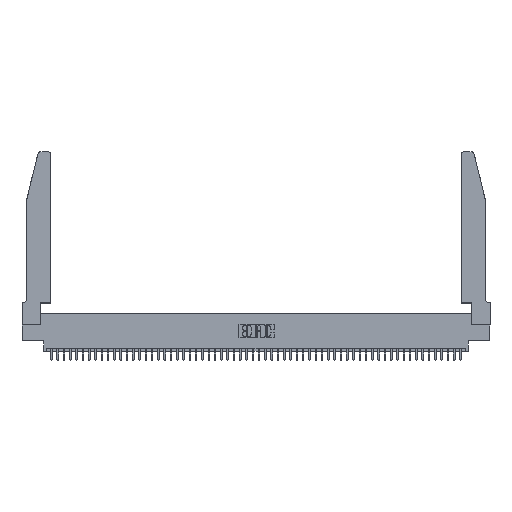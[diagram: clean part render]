
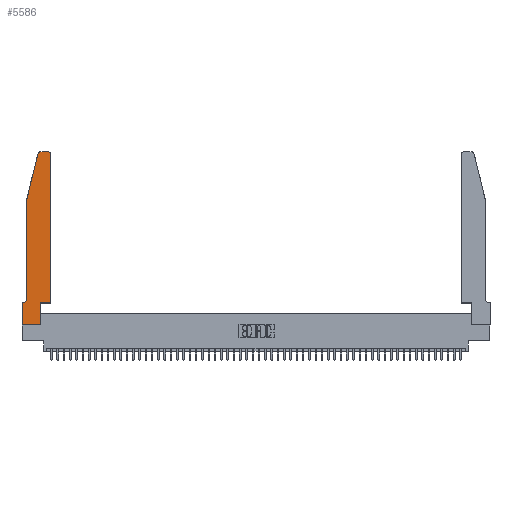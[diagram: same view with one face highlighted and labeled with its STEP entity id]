
A CAD part, top view. The second image highlights one B-rep face of the part: STEP entity #5586.
In plain terms, the highlighted planar face has unit normal (0, 0, 1).
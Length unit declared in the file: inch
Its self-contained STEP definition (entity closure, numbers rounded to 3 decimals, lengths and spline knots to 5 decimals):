
#58 = DIRECTION ( 'NONE',  ( 0., 0., 1. ) ) ;
#455 = VECTOR ( 'NONE', #43000, 39.37008 ) ;
#641 = VERTEX_POINT ( 'NONE', #29714 ) ;
#817 = CARTESIAN_POINT ( 'NONE',  ( 0.0755, 2., 0.37 ) ) ;
#2398 = EDGE_CURVE ( 'NONE', #641, #36479, #14091, .T. ) ;
#4239 = CARTESIAN_POINT ( 'NONE',  ( 0.0755, 2., 0.37 ) ) ;
#4984 = ORIENTED_EDGE ( 'NONE', *, *, #37938, .T. ) ;
#5417 = VERTEX_POINT ( 'NONE', #32110 ) ;
#5586 = ADVANCED_FACE ( 'NONE', ( #47401 ), #8247, .T. ) ;
#5606 = VERTEX_POINT ( 'NONE', #4239 ) ;
#5927 = ORIENTED_EDGE ( 'NONE', *, *, #8302, .T. ) ;
#6263 = VERTEX_POINT ( 'NONE', #37422 ) ;
#6412 = DIRECTION ( 'NONE',  ( 0., -1., 0. ) ) ;
#7807 = VECTOR ( 'NONE', #10816, 39.37008 ) ;
#8247 = PLANE ( 'NONE',  #50703 ) ;
#8302 = EDGE_CURVE ( 'NONE', #5606, #12480, #20822, .T. ) ;
#8581 = EDGE_CURVE ( 'NONE', #42707, #641, #31118, .T. ) ;
#9226 = VECTOR ( 'NONE', #50656, 39.37008 ) ;
#10210 = DIRECTION ( 'NONE',  ( 0., 0., -1. ) ) ;
#10615 = CARTESIAN_POINT ( 'NONE',  ( 0.0755, 0.42, 0.37 ) ) ;
#10816 = DIRECTION ( 'NONE',  ( 1., 0., 0. ) ) ;
#12480 = VERTEX_POINT ( 'NONE', #10615 ) ;
#13121 = CARTESIAN_POINT ( 'NONE',  ( 0.0755, 0.35, 0.37 ) ) ;
#13303 = CARTESIAN_POINT ( 'NONE',  ( 0.2865, 0.35, 0.37 ) ) ;
#13602 = EDGE_LOOP ( 'NONE', ( #52687, #4984, #48419, #5927, #28442, #44120, #22112, #52174, #36251, #24450, #34792, #44723 ) ) ;
#14091 = LINE ( 'NONE', #51625, #45785 ) ;
#14487 = DIRECTION ( 'NONE',  ( 0., 1., 0. ) ) ;
#14609 = VERTEX_POINT ( 'NONE', #30704 ) ;
#15669 = EDGE_CURVE ( 'NONE', #36479, #23356, #40565, .T. ) ;
#17044 = CARTESIAN_POINT ( 'NONE',  ( 0.0755, 2., 0.37 ) ) ;
#17643 = EDGE_CURVE ( 'NONE', #41685, #5606, #53184, .T. ) ;
#18992 = EDGE_CURVE ( 'NONE', #5417, #22556, #51760, .T. ) ;
#20329 = VECTOR ( 'NONE', #21215, 39.37008 ) ;
#20747 = CARTESIAN_POINT ( 'NONE',  ( 0., 0.35, 0.37 ) ) ;
#20822 = LINE ( 'NONE', #817, #31774 ) ;
#20905 = CARTESIAN_POINT ( 'NONE',  ( 0.25487, 2.72718, 0.37 ) ) ;
#20945 = CARTESIAN_POINT ( 'NONE',  ( 0.284, 2.72, 0.37 ) ) ;
#21215 = DIRECTION ( 'NONE',  ( -0.239, -0.971, 0. ) ) ;
#21422 = DIRECTION ( 'NONE',  ( 0., 0., 1. ) ) ;
#21549 = LINE ( 'NONE', #46560, #9226 ) ;
#22112 = ORIENTED_EDGE ( 'NONE', *, *, #18992, .T. ) ;
#22556 = VERTEX_POINT ( 'NONE', #28839 ) ;
#22835 = CARTESIAN_POINT ( 'NONE',  ( 0.4505, 2.72, 0.37 ) ) ;
#22876 = EDGE_CURVE ( 'NONE', #12480, #6263, #52222, .T. ) ;
#23356 = VERTEX_POINT ( 'NONE', #46453 ) ;
#23454 = EDGE_CURVE ( 'NONE', #23356, #14609, #33487, .T. ) ;
#24450 = ORIENTED_EDGE ( 'NONE', *, *, #8581, .T. ) ;
#25080 = DIRECTION ( 'NONE',  ( 1., 0., 0. ) ) ;
#27059 = VECTOR ( 'NONE', #46171, 39.37008 ) ;
#27079 = EDGE_CURVE ( 'NONE', #22556, #49435, #21549, .T. ) ;
#27228 = CARTESIAN_POINT ( 'NONE',  ( 0., 0., 0.37 ) ) ;
#27248 = CARTESIAN_POINT ( 'NONE',  ( 0.4505, 0.35, 0.37 ) ) ;
#28441 = DIRECTION ( 'NONE',  ( 0., 1., 0. ) ) ;
#28442 = ORIENTED_EDGE ( 'NONE', *, *, #22876, .T. ) ;
#28558 = VECTOR ( 'NONE', #6412, 39.37008 ) ;
#28839 = CARTESIAN_POINT ( 'NONE',  ( 0., 0., 0.37 ) ) ;
#29033 = DIRECTION ( 'NONE',  ( 1., 0., 0. ) ) ;
#29714 = CARTESIAN_POINT ( 'NONE',  ( 0.4505, 0.35, 0.37 ) ) ;
#29892 = LINE ( 'NONE', #40903, #43458 ) ;
#30704 = CARTESIAN_POINT ( 'NONE',  ( 0.284, 2.75, 0.37 ) ) ;
#31118 = LINE ( 'NONE', #27248, #7807 ) ;
#31774 = VECTOR ( 'NONE', #37888, 39.37008 ) ;
#32110 = CARTESIAN_POINT ( 'NONE',  ( 0., 0.35, 0.37 ) ) ;
#32181 = EDGE_CURVE ( 'NONE', #6263, #5417, #48984, .T. ) ;
#32768 = AXIS2_PLACEMENT_3D ( 'NONE', #46135, #21422, #50231 ) ;
#33487 = LINE ( 'NONE', #38840, #455 ) ;
#33744 = AXIS2_PLACEMENT_3D ( 'NONE', #34917, #10210, #39082 ) ;
#34782 = AXIS2_PLACEMENT_3D ( 'NONE', #20945, #49758, #25080 ) ;
#34792 = ORIENTED_EDGE ( 'NONE', *, *, #2398, .T. ) ;
#34917 = CARTESIAN_POINT ( 'NONE',  ( 0.0055, 0.42, 0.37 ) ) ;
#36251 = ORIENTED_EDGE ( 'NONE', *, *, #50395, .T. ) ;
#36479 = VERTEX_POINT ( 'NONE', #22835 ) ;
#37422 = CARTESIAN_POINT ( 'NONE',  ( 0.0055, 0.35, 0.37 ) ) ;
#37888 = DIRECTION ( 'NONE',  ( 0., -1., 0. ) ) ;
#37938 = EDGE_CURVE ( 'NONE', #14609, #41685, #52615, .T. ) ;
#38840 = CARTESIAN_POINT ( 'NONE',  ( 0.2605, 2.75, 0.37 ) ) ;
#39082 = DIRECTION ( 'NONE',  ( -1., 0., 0. ) ) ;
#40565 = CIRCLE ( 'NONE', #32768, 0.03 ) ;
#40903 = CARTESIAN_POINT ( 'NONE',  ( 0.2865, 0.35, 0.37 ) ) ;
#41685 = VERTEX_POINT ( 'NONE', #20905 ) ;
#42707 = VERTEX_POINT ( 'NONE', #13303 ) ;
#43000 = DIRECTION ( 'NONE',  ( -1., 0., 0. ) ) ;
#43458 = VECTOR ( 'NONE', #28441, 39.37008 ) ;
#44120 = ORIENTED_EDGE ( 'NONE', *, *, #32181, .T. ) ;
#44723 = ORIENTED_EDGE ( 'NONE', *, *, #15669, .T. ) ;
#45785 = VECTOR ( 'NONE', #14487, 39.37008 ) ;
#46135 = CARTESIAN_POINT ( 'NONE',  ( 0.4205, 2.72, 0.37 ) ) ;
#46171 = DIRECTION ( 'NONE',  ( -1., 0., 0. ) ) ;
#46453 = CARTESIAN_POINT ( 'NONE',  ( 0.4205, 2.75, 0.37 ) ) ;
#46560 = CARTESIAN_POINT ( 'NONE',  ( 0., 0., 0.37 ) ) ;
#47401 = FACE_OUTER_BOUND ( 'NONE', #13602, .T. ) ;
#48419 = ORIENTED_EDGE ( 'NONE', *, *, #17643, .T. ) ;
#48984 = LINE ( 'NONE', #13121, #27059 ) ;
#49093 = CARTESIAN_POINT ( 'NONE',  ( 0.2865, 0., 0.37 ) ) ;
#49435 = VERTEX_POINT ( 'NONE', #49093 ) ;
#49758 = DIRECTION ( 'NONE',  ( 0., 0., 1. ) ) ;
#50231 = DIRECTION ( 'NONE',  ( 1., 0., 0. ) ) ;
#50395 = EDGE_CURVE ( 'NONE', #49435, #42707, #29892, .T. ) ;
#50656 = DIRECTION ( 'NONE',  ( 1., 0., 0. ) ) ;
#50703 = AXIS2_PLACEMENT_3D ( 'NONE', #20747, #58, #29033 ) ;
#51625 = CARTESIAN_POINT ( 'NONE',  ( 0.4505, 0.35, 0.37 ) ) ;
#51760 = LINE ( 'NONE', #27228, #28558 ) ;
#52174 = ORIENTED_EDGE ( 'NONE', *, *, #27079, .T. ) ;
#52222 = CIRCLE ( 'NONE', #33744, 0.07 ) ;
#52615 = CIRCLE ( 'NONE', #34782, 0.03 ) ;
#52687 = ORIENTED_EDGE ( 'NONE', *, *, #23454, .T. ) ;
#53184 = LINE ( 'NONE', #17044, #20329 ) ;
